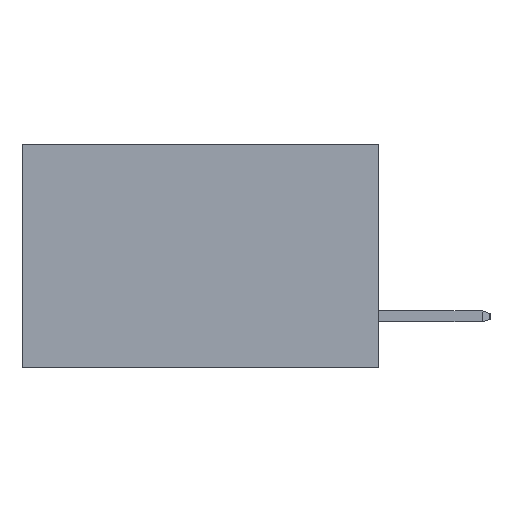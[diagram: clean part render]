
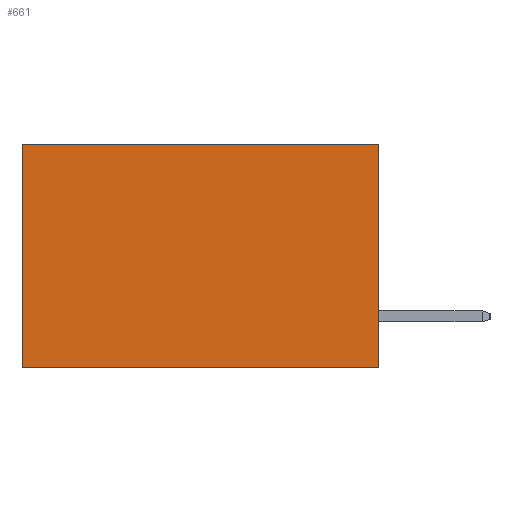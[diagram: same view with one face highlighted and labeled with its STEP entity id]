
A CAD part, left-side view. The second image highlights one B-rep face of the part: STEP entity #661.
In plain terms, the highlighted planar face has unit normal (-1, 0, 0).
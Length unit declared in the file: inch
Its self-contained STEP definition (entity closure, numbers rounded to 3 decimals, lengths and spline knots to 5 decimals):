
#225 = AXIS2_PLACEMENT_3D ( 'NONE', #17871, #1397, #2707 ) ;
#661 = ADVANCED_FACE ( 'NONE', ( #16915 ), #17945, .F. ) ;
#1397 = DIRECTION ( 'NONE',  ( 1., 0., 0. ) ) ;
#1979 = EDGE_CURVE ( 'NONE', #12258, #10166, #2027, .T. ) ;
#2027 = LINE ( 'NONE', #19426, #15497 ) ;
#2252 = EDGE_CURVE ( 'NONE', #16638, #9832, #9273, .T. ) ;
#2598 = EDGE_LOOP ( 'NONE', ( #8355, #14086, #18636, #14620 ) ) ;
#2707 = DIRECTION ( 'NONE',  ( 0., 0., -1. ) ) ;
#3869 = DIRECTION ( 'NONE',  ( 0., 1., 0. ) ) ;
#4193 = EDGE_CURVE ( 'NONE', #12258, #16638, #22387, .T. ) ;
#4936 = EDGE_CURVE ( 'NONE', #10166, #9832, #20572, .T. ) ;
#6318 = CARTESIAN_POINT ( 'NONE',  ( 0.277, 0., -0.37 ) ) ;
#8355 = ORIENTED_EDGE ( 'NONE', *, *, #4936, .T. ) ;
#9273 = LINE ( 'NONE', #22038, #17908 ) ;
#9832 = VERTEX_POINT ( 'NONE', #17603 ) ;
#9912 = DIRECTION ( 'NONE',  ( 0., 0., -1. ) ) ;
#10166 = VERTEX_POINT ( 'NONE', #15062 ) ;
#11550 = DIRECTION ( 'NONE',  ( 0., 1., 0. ) ) ;
#12175 = DIRECTION ( 'NONE',  ( 0., 0., -1. ) ) ;
#12258 = VERTEX_POINT ( 'NONE', #14421 ) ;
#14086 = ORIENTED_EDGE ( 'NONE', *, *, #2252, .F. ) ;
#14421 = CARTESIAN_POINT ( 'NONE',  ( 0.277, 0., 0. ) ) ;
#14620 = ORIENTED_EDGE ( 'NONE', *, *, #1979, .T. ) ;
#15062 = CARTESIAN_POINT ( 'NONE',  ( 0.277, 0.59, 0. ) ) ;
#15497 = VECTOR ( 'NONE', #3869, 39.37008 ) ;
#16089 = VECTOR ( 'NONE', #12175, 39.37008 ) ;
#16638 = VERTEX_POINT ( 'NONE', #20838 ) ;
#16915 = FACE_OUTER_BOUND ( 'NONE', #2598, .T. ) ;
#17603 = CARTESIAN_POINT ( 'NONE',  ( 0.277, 0.59, -0.37 ) ) ;
#17871 = CARTESIAN_POINT ( 'NONE',  ( 0.277, 0., -0.37 ) ) ;
#17908 = VECTOR ( 'NONE', #11550, 39.37008 ) ;
#17945 = PLANE ( 'NONE',  #225 ) ;
#18537 = VECTOR ( 'NONE', #9912, 39.37008 ) ;
#18636 = ORIENTED_EDGE ( 'NONE', *, *, #4193, .F. ) ;
#19426 = CARTESIAN_POINT ( 'NONE',  ( 0.277, 0., 0. ) ) ;
#20572 = LINE ( 'NONE', #22119, #16089 ) ;
#20838 = CARTESIAN_POINT ( 'NONE',  ( 0.277, 0., -0.37 ) ) ;
#22038 = CARTESIAN_POINT ( 'NONE',  ( 0.277, 0., -0.37 ) ) ;
#22119 = CARTESIAN_POINT ( 'NONE',  ( 0.277, 0.59, -0.37 ) ) ;
#22387 = LINE ( 'NONE', #6318, #18537 ) ;
